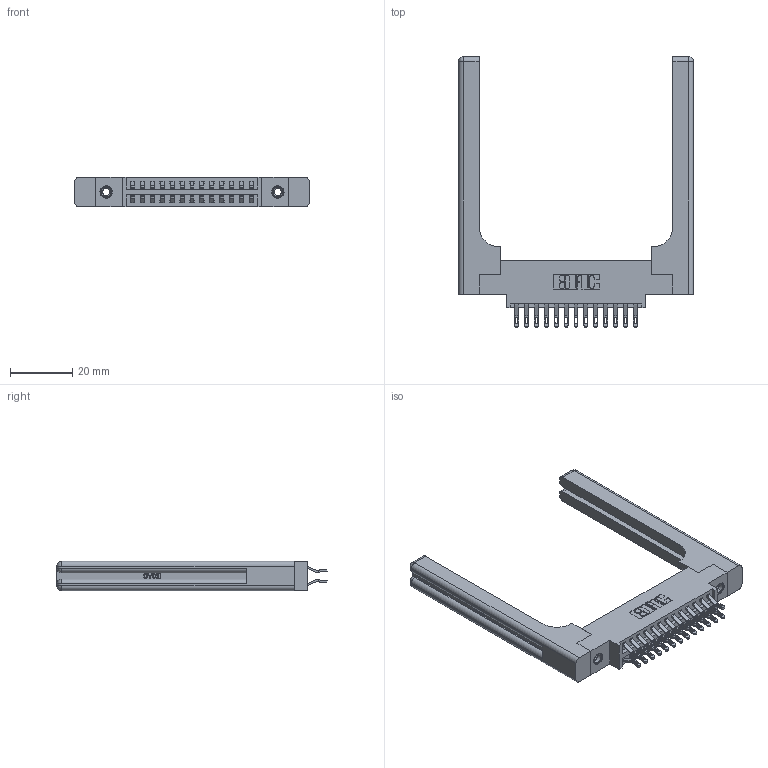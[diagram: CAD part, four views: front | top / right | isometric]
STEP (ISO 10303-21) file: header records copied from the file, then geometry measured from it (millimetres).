
FILE_DESCRIPTION (( 'STEP AP203' ), '1' );
FILE_NAME ('346-026-555-858.STEP', '2022-05-19T02:25:34', ( '' ), ( '' ), 'SwSTEP 2.0', 'SolidWorks 2020', '' );
FILE_SCHEMA (( 'CONFIG_CONTROL_DESIGN' ));
Length unit declared in the file: inch
Products named in the file (5): 346-026-555-858; 346 Part_0.170 Offset - 0.156 Dia-TH; 346-220-058_345-220-058; 345-292-001_555 Tail; 345-250-001_345-250-001-102
Assembly tree (31 placements, depth 2):
  346-026-555-858
    346 Part_0.170 Offset - 0.156 Dia-TH
    345-292-001_555 Tail  x26
    345-250-001_345-250-001-102  x2
    346-220-058_345-220-058  x2
Bounding box: 75.34 x 86.74 x 9.4 mm (x, y, z)
Volume: 14517.9 mm3; surface area: 14654.5 mm2
Topology: 31 solids, 31 shells, 1904 faces, 5801 edges, 3846 vertices
Faces by surface type: plane 1100, cylinder 744, bspline 36, cone 12, sphere 8, torus 4
Entity records: 18444 total; most frequent: CARTESIAN_POINT 4129, ORIENTED_EDGE 2828, DIRECTION 2590, EDGE_CURVE 1414, LINE 1118, VECTOR 1118, VERTEX_POINT 934, AXIS2_PLACEMENT_3D 736
